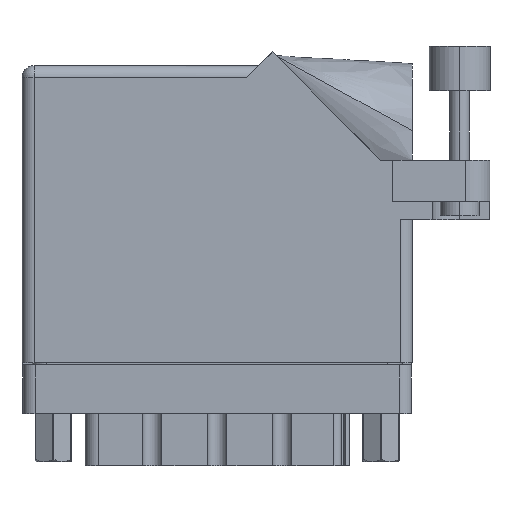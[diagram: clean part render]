
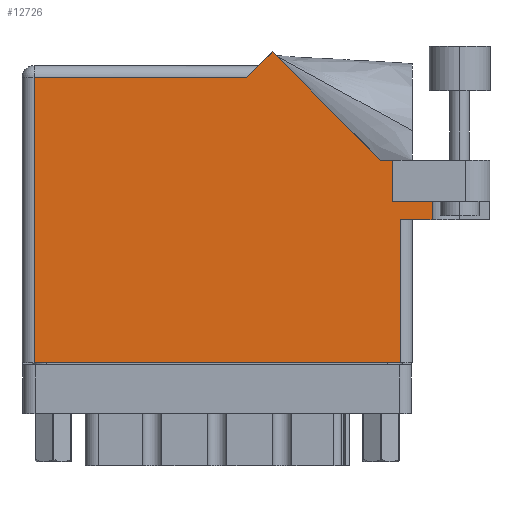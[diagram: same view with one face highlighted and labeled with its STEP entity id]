
A CAD part, front view. The second image highlights one B-rep face of the part: STEP entity #12726.
In plain terms, the highlighted face is planar.
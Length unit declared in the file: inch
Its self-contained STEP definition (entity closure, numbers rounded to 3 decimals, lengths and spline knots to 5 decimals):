
#252 = VECTOR ( 'NONE', #10432, 39.37008 ) ;
#484 = DIRECTION ( 'NONE',  ( -0.707, 0.707, 0. ) ) ;
#1227 = CARTESIAN_POINT ( 'NONE',  ( 1.91, 0.831, 0. ) ) ;
#1308 = LINE ( 'NONE', #40499, #26884 ) ;
#1761 = DIRECTION ( 'NONE',  ( 0., 1., 0. ) ) ;
#1810 = VERTEX_POINT ( 'NONE', #24289 ) ;
#2756 = CARTESIAN_POINT ( 'NONE',  ( 1.28771, 1.60071, 0. ) ) ;
#3064 = ORIENTED_EDGE ( 'NONE', *, *, #45499, .T. ) ;
#3339 = CARTESIAN_POINT ( 'NONE',  ( 1.948, 0.737, 0. ) ) ;
#3651 = ORIENTED_EDGE ( 'NONE', *, *, #26416, .T. ) ;
#3969 = LINE ( 'NONE', #42664, #49855 ) ;
#4965 = VECTOR ( 'NONE', #44279, 39.37008 ) ;
#5825 = VERTEX_POINT ( 'NONE', #9470 ) ;
#6902 = LINE ( 'NONE', #49644, #43959 ) ;
#7433 = VERTEX_POINT ( 'NONE', #2756 ) ;
#9315 = VECTOR ( 'NONE', #484, 39.37008 ) ;
#9470 = CARTESIAN_POINT ( 'NONE',  ( 0.062, 0., 0. ) ) ;
#9927 = LINE ( 'NONE', #28753, #4965 ) ;
#10432 = DIRECTION ( 'NONE',  ( -0.707, -0.707, 0. ) ) ;
#10802 = ORIENTED_EDGE ( 'NONE', *, *, #42839, .F. ) ;
#11886 = LINE ( 'NONE', #34630, #25281 ) ;
#11899 = ORIENTED_EDGE ( 'NONE', *, *, #33281, .T. ) ;
#12705 = CARTESIAN_POINT ( 'NONE',  ( 1.948, 0.737, 0. ) ) ;
#12726 = ADVANCED_FACE ( 'NONE', ( #40555 ), #37005, .F. ) ;
#12951 = LINE ( 'NONE', #12705, #20481 ) ;
#14741 = CARTESIAN_POINT ( 'NONE',  ( 1.217, 1.53, 0. ) ) ;
#14779 = VERTEX_POINT ( 'NONE', #32860 ) ;
#14941 = EDGE_CURVE ( 'NONE', #23659, #5825, #6902, .T. ) ;
#14966 = ORIENTED_EDGE ( 'NONE', *, *, #30901, .T. ) ;
#16203 = LINE ( 'NONE', #35795, #26588 ) ;
#16975 = CARTESIAN_POINT ( 'NONE',  ( 1.84442, 1.044, 0. ) ) ;
#19452 = VERTEX_POINT ( 'NONE', #3339 ) ;
#19707 = VERTEX_POINT ( 'NONE', #31322 ) ;
#20074 = CARTESIAN_POINT ( 'NONE',  ( 0.062, 1.468, 0. ) ) ;
#20277 = VERTEX_POINT ( 'NONE', #16975 ) ;
#20481 = VECTOR ( 'NONE', #1761, 39.37008 ) ;
#23659 = VERTEX_POINT ( 'NONE', #20074 ) ;
#24289 = CARTESIAN_POINT ( 'NONE',  ( 1.155, 1.468, 0. ) ) ;
#25281 = VECTOR ( 'NONE', #38460, 39.37008 ) ;
#25524 = EDGE_CURVE ( 'NONE', #5825, #14779, #16203, .T. ) ;
#26416 = EDGE_CURVE ( 'NONE', #40384, #20277, #1308, .T. ) ;
#26588 = VECTOR ( 'NONE', #47516, 39.37008 ) ;
#26699 = ORIENTED_EDGE ( 'NONE', *, *, #41441, .T. ) ;
#26818 = VECTOR ( 'NONE', #34974, 39.37008 ) ;
#26884 = VECTOR ( 'NONE', #48397, 39.37008 ) ;
#27384 = EDGE_CURVE ( 'NONE', #19707, #38273, #9927, .T. ) ;
#27862 = ORIENTED_EDGE ( 'NONE', *, *, #31408, .T. ) ;
#28753 = CARTESIAN_POINT ( 'NONE',  ( 2.1115, 1.16177, 0. ) ) ;
#28968 = EDGE_CURVE ( 'NONE', #19452, #38273, #11886, .T. ) ;
#29631 = DIRECTION ( 'NONE',  ( -1., 0., 0. ) ) ;
#29976 = CARTESIAN_POINT ( 'NONE',  ( 1.91, 1.044, 0. ) ) ;
#30901 = EDGE_CURVE ( 'NONE', #7433, #1810, #33836, .T. ) ;
#31213 = DIRECTION ( 'NONE',  ( -1., 0., 0. ) ) ;
#31322 = CARTESIAN_POINT ( 'NONE',  ( 2.1115, 0.831, 0. ) ) ;
#31408 = EDGE_CURVE ( 'NONE', #1810, #23659, #3969, .T. ) ;
#31771 = CARTESIAN_POINT ( 'NONE',  ( 1.84442, 1.044, 0. ) ) ;
#32860 = CARTESIAN_POINT ( 'NONE',  ( 1.948, 0., 0. ) ) ;
#33281 = EDGE_CURVE ( 'NONE', #20277, #7433, #35344, .T. ) ;
#33836 = LINE ( 'NONE', #14741, #252 ) ;
#34630 = CARTESIAN_POINT ( 'NONE',  ( 2.01, 0.737, 0. ) ) ;
#34974 = DIRECTION ( 'NONE',  ( 1., 0., 0. ) ) ;
#35344 = LINE ( 'NONE', #31771, #9315 ) ;
#35795 = CARTESIAN_POINT ( 'NONE',  ( 0., 0., 0. ) ) ;
#35915 = ORIENTED_EDGE ( 'NONE', *, *, #28968, .T. ) ;
#36278 = CARTESIAN_POINT ( 'NONE',  ( 2.1115, 0.737, 0. ) ) ;
#36403 = VERTEX_POINT ( 'NONE', #1227 ) ;
#36871 = ORIENTED_EDGE ( 'NONE', *, *, #27384, .F. ) ;
#37005 = PLANE ( 'NONE',  #39214 ) ;
#37260 = DIRECTION ( 'NONE',  ( 0., 0., -1. ) ) ;
#38273 = VERTEX_POINT ( 'NONE', #36278 ) ;
#38460 = DIRECTION ( 'NONE',  ( 1., 0., 0. ) ) ;
#39052 = LINE ( 'NONE', #46208, #26818 ) ;
#39214 = AXIS2_PLACEMENT_3D ( 'NONE', #44121, #37260, #29631 ) ;
#40384 = VERTEX_POINT ( 'NONE', #29976 ) ;
#40499 = CARTESIAN_POINT ( 'NONE',  ( 2.41, 1.044, 0. ) ) ;
#40512 = ORIENTED_EDGE ( 'NONE', *, *, #14941, .T. ) ;
#40555 = FACE_OUTER_BOUND ( 'NONE', #45868, .T. ) ;
#41441 = EDGE_CURVE ( 'NONE', #36403, #40384, #49767, .T. ) ;
#42664 = CARTESIAN_POINT ( 'NONE',  ( 0., 1.468, 0. ) ) ;
#42839 = EDGE_CURVE ( 'NONE', #36403, #19707, #39052, .T. ) ;
#43959 = VECTOR ( 'NONE', #45578, 39.37008 ) ;
#44121 = CARTESIAN_POINT ( 'NONE',  ( 0., 1.53, 0. ) ) ;
#44279 = DIRECTION ( 'NONE',  ( 0., -1., 0. ) ) ;
#45499 = EDGE_CURVE ( 'NONE', #14779, #19452, #12951, .T. ) ;
#45578 = DIRECTION ( 'NONE',  ( 0., -1., 0. ) ) ;
#45868 = EDGE_LOOP ( 'NONE', ( #46736, #3064, #35915, #36871, #10802, #26699, #3651, #11899, #14966, #27862, #40512 ) ) ;
#46208 = CARTESIAN_POINT ( 'NONE',  ( 1.91, 0.831, 0. ) ) ;
#46697 = DIRECTION ( 'NONE',  ( 0., 1., 0. ) ) ;
#46736 = ORIENTED_EDGE ( 'NONE', *, *, #25524, .T. ) ;
#46936 = CARTESIAN_POINT ( 'NONE',  ( 1.91, 0.831, 0. ) ) ;
#47516 = DIRECTION ( 'NONE',  ( 1., 0., 0. ) ) ;
#48397 = DIRECTION ( 'NONE',  ( -1., 0., 0. ) ) ;
#49644 = CARTESIAN_POINT ( 'NONE',  ( 0.062, 0., 0. ) ) ;
#49767 = LINE ( 'NONE', #46936, #50293 ) ;
#49855 = VECTOR ( 'NONE', #31213, 39.37008 ) ;
#50293 = VECTOR ( 'NONE', #46697, 39.37008 ) ;
